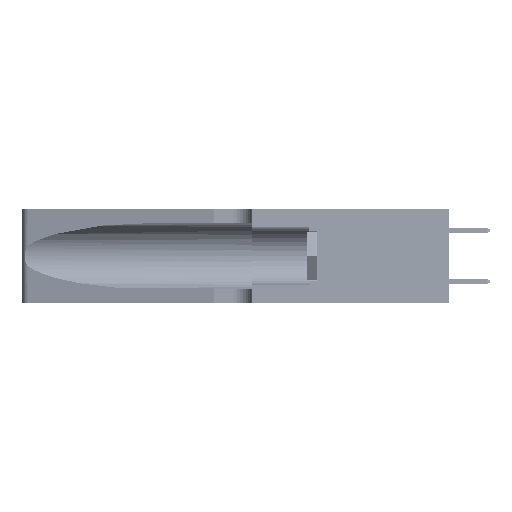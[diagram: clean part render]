
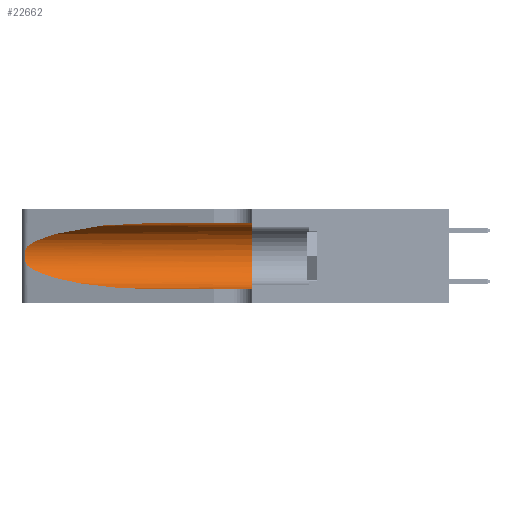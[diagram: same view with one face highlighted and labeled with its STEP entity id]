
A CAD part, left-side view. The second image highlights one B-rep face of the part: STEP entity #22662.
In plain terms, the highlighted cylindrical face has radius 3.308 mm (diameter 6.617 mm), a partial arc.
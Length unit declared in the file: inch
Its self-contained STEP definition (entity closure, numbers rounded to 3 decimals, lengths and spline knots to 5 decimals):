
#127 = CARTESIAN_POINT ( 'NONE',  ( 0.18966, 0.96281, 0.31525 ) ) ;
#707 = ORIENTED_EDGE ( 'NONE', *, *, #7061, .T. ) ;
#1050 = CYLINDRICAL_SURFACE ( 'NONE', #9295, 0.13025 ) ;
#2279 = FACE_OUTER_BOUND ( 'NONE', #49194, .T. ) ;
#2919 = VERTEX_POINT ( 'NONE', #35801 ) ;
#3075 = ORIENTED_EDGE ( 'NONE', *, *, #43091, .T. ) ;
#3506 = CARTESIAN_POINT ( 'NONE',  ( 0.25639, 1.23184, 0.21858 ) ) ;
#3718 = VERTEX_POINT ( 'NONE', #8474 ) ;
#4155 = CARTESIAN_POINT ( 'NONE',  ( 0.25487, 1.22718, 0.22369 ) ) ;
#4315 = DIRECTION ( 'NONE',  ( 0., 1., 0. ) ) ;
#5175 = EDGE_CURVE ( 'NONE', #48116, #2919, #51474, .T. ) ;
#5229 = CARTESIAN_POINT ( 'NONE',  ( 0.1305, 0.72297, 0.05475 ) ) ;
#7061 = EDGE_CURVE ( 'NONE', #45883, #2919, #39023, .T. ) ;
#7151 = VECTOR ( 'NONE', #13719, 39.37008 ) ;
#7478 = LINE ( 'NONE', #19721, #26257 ) ;
#7568 = CARTESIAN_POINT ( 'NONE',  ( 0.25854, 1.2359, 0.20912 ) ) ;
#7797 = DIRECTION ( 'NONE',  ( 0., -1., 0. ) ) ;
#8188 = EDGE_CURVE ( 'NONE', #44306, #35094, #8784, .T. ) ;
#8474 = CARTESIAN_POINT ( 'NONE',  ( 0.25487, 1.22718, 0.14631 ) ) ;
#8784 =( BOUNDED_CURVE ( )  B_SPLINE_CURVE ( 3, ( #47873, #127, #28163, #4155 ),
 .UNSPECIFIED., .F., .F. ) 
 B_SPLINE_CURVE_WITH_KNOTS ( ( 4, 4 ),
 ( 1.5708, 2.84003 ),
 .UNSPECIFIED. ) 
 CURVE ( )  GEOMETRIC_REPRESENTATION_ITEM ( )  RATIONAL_B_SPLINE_CURVE ( ( 1., 0.87, 0.87, 1. ) ) 
 REPRESENTATION_ITEM ( '' )  );
#9295 = AXIS2_PLACEMENT_3D ( 'NONE', #17488, #49240, #25502 ) ;
#11609 = CARTESIAN_POINT ( 'NONE',  ( 0.26075, 1.23896, 0.19203 ) ) ;
#13719 = DIRECTION ( 'NONE',  ( 0., -1., 0. ) ) ;
#14804 = ORIENTED_EDGE ( 'NONE', *, *, #5175, .F. ) ;
#15675 = CARTESIAN_POINT ( 'NONE',  ( 0.26017, 1.23833, 0.17102 ) ) ;
#17203 = CARTESIAN_POINT ( 'NONE',  ( 0.2373, 1.15595, 0.08982 ) ) ;
#17488 = CARTESIAN_POINT ( 'NONE',  ( 0.1305, 1.61858, 0.185 ) ) ;
#17609 = EDGE_CURVE ( 'NONE', #44306, #48116, #7478, .T. ) ;
#18291 = CARTESIAN_POINT ( 'NONE',  ( 0.1305, 0.35, 0.31525 ) ) ;
#19661 = CARTESIAN_POINT ( 'NONE',  ( 0.25789, 1.23486, 0.15765 ) ) ;
#19721 = CARTESIAN_POINT ( 'NONE',  ( 0.1305, 1.61858, 0.31525 ) ) ;
#22662 = ADVANCED_FACE ( 'NONE', ( #2279 ), #1050, .F. ) ;
#23670 = CARTESIAN_POINT ( 'NONE',  ( 0.25555, 1.22993, 0.14849 ) ) ;
#25101 = CARTESIAN_POINT ( 'NONE',  ( 0.1305, 0.72297, 0.31525 ) ) ;
#25190 = AXIS2_PLACEMENT_3D ( 'NONE', #28312, #4315, #32276 ) ;
#25502 = DIRECTION ( 'NONE',  ( 0., 0., -1. ) ) ;
#26257 = VECTOR ( 'NONE', #7797, 39.37008 ) ;
#27526 = CARTESIAN_POINT ( 'NONE',  ( 0.25555, 1.22994, 0.2215 ) ) ;
#28163 = CARTESIAN_POINT ( 'NONE',  ( 0.2373, 1.15595, 0.28018 ) ) ;
#28312 = CARTESIAN_POINT ( 'NONE',  ( 0.1305, 0.35, 0.185 ) ) ;
#28982 = B_SPLINE_CURVE_WITH_KNOTS ( 'NONE', 3,
 ( #51215, #27526, #3506, #31493, #7568, #35519, #11609, #39530, #15675, #43480, #19661, #47433, #23670, #51392 ),
 .UNSPECIFIED., .F., .F.,
 ( 4, 2, 2, 2, 2, 2, 4 ),
 ( 0., 0.00027, 0.00053, 0.00107, 0.0016, 0.00187, 0.00214 ),
 .UNSPECIFIED. ) ;
#29196 = CARTESIAN_POINT ( 'NONE',  ( 0.18966, 0.96281, 0.05475 ) ) ;
#31493 = CARTESIAN_POINT ( 'NONE',  ( 0.25787, 1.23484, 0.2124 ) ) ;
#32140 = ORIENTED_EDGE ( 'NONE', *, *, #8188, .T. ) ;
#32276 = DIRECTION ( 'NONE',  ( 0., 0., 1. ) ) ;
#33593 = CARTESIAN_POINT ( 'NONE',  ( 0.1305, 1.61858, 0.05475 ) ) ;
#35094 = VERTEX_POINT ( 'NONE', #48151 ) ;
#35519 = CARTESIAN_POINT ( 'NONE',  ( 0.26018, 1.23835, 0.19895 ) ) ;
#35801 = CARTESIAN_POINT ( 'NONE',  ( 0.1305, 0.35, 0.05475 ) ) ;
#38200 =( BOUNDED_CURVE ( )  B_SPLINE_CURVE ( 3, ( #44988, #17203, #29196, #5229 ),
 .UNSPECIFIED., .F., .T. ) 
 B_SPLINE_CURVE_WITH_KNOTS ( ( 4, 4 ),
 ( 3.44316, 4.71239 ),
 .UNSPECIFIED. ) 
 CURVE ( )  GEOMETRIC_REPRESENTATION_ITEM ( )  RATIONAL_B_SPLINE_CURVE ( ( 1., 0.87, 0.87, 1. ) ) 
 REPRESENTATION_ITEM ( '' )  );
#39023 = LINE ( 'NONE', #33593, #7151 ) ;
#39530 = CARTESIAN_POINT ( 'NONE',  ( 0.26075, 1.23896, 0.178 ) ) ;
#41308 = ORIENTED_EDGE ( 'NONE', *, *, #48344, .T. ) ;
#42332 = CARTESIAN_POINT ( 'NONE',  ( 0.1305, 0.72297, 0.05475 ) ) ;
#43091 = EDGE_CURVE ( 'NONE', #3718, #45883, #38200, .T. ) ;
#43480 = CARTESIAN_POINT ( 'NONE',  ( 0.25856, 1.23593, 0.16098 ) ) ;
#44306 = VERTEX_POINT ( 'NONE', #25101 ) ;
#44535 = ORIENTED_EDGE ( 'NONE', *, *, #17609, .F. ) ;
#44988 = CARTESIAN_POINT ( 'NONE',  ( 0.25487, 1.22718, 0.14631 ) ) ;
#45883 = VERTEX_POINT ( 'NONE', #42332 ) ;
#47433 = CARTESIAN_POINT ( 'NONE',  ( 0.25639, 1.23186, 0.15144 ) ) ;
#47873 = CARTESIAN_POINT ( 'NONE',  ( 0.1305, 0.72297, 0.31525 ) ) ;
#48116 = VERTEX_POINT ( 'NONE', #18291 ) ;
#48151 = CARTESIAN_POINT ( 'NONE',  ( 0.25487, 1.22718, 0.22369 ) ) ;
#48344 = EDGE_CURVE ( 'NONE', #35094, #3718, #28982, .T. ) ;
#49194 = EDGE_LOOP ( 'NONE', ( #32140, #41308, #3075, #707, #14804, #44535 ) ) ;
#49240 = DIRECTION ( 'NONE',  ( 0., -1., 0. ) ) ;
#51215 = CARTESIAN_POINT ( 'NONE',  ( 0.25487, 1.22718, 0.22369 ) ) ;
#51392 = CARTESIAN_POINT ( 'NONE',  ( 0.25487, 1.22718, 0.14631 ) ) ;
#51474 = CIRCLE ( 'NONE', #25190, 0.13025 ) ;
